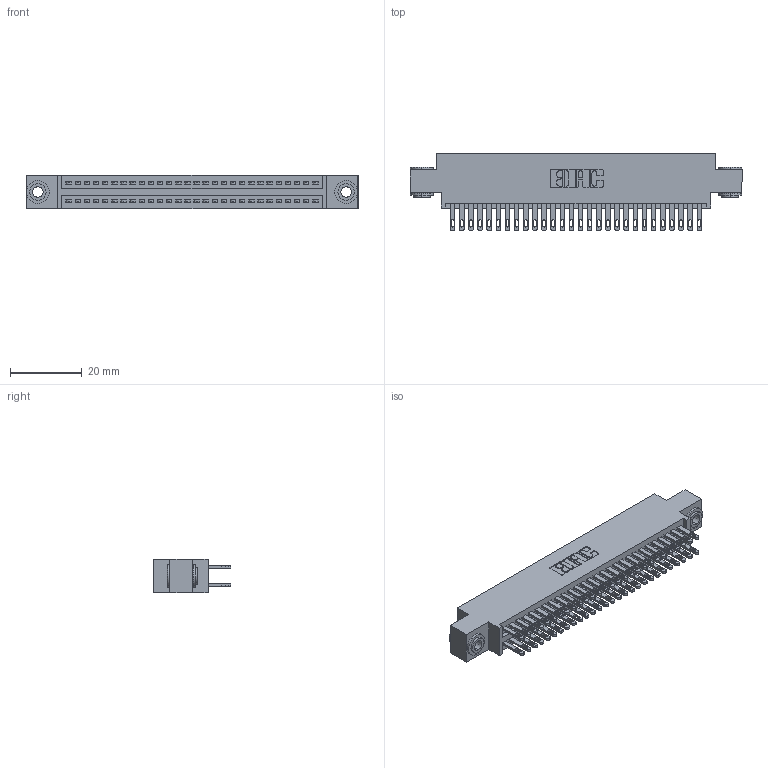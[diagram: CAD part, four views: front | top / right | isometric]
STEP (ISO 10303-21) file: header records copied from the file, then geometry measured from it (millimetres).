
FILE_DESCRIPTION (( 'STEP AP203' ), '1' );
FILE_NAME ('895-056-500-803.STEP', '2020-09-27T16:11:26', ( '' ), ( '' ), 'SwSTEP 2.0', 'SolidWorks 2020', '' );
FILE_SCHEMA (( 'CONFIG_CONTROL_DESIGN' ));
Length unit declared in the file: inch
Products named in the file (4): 345-292-001_345-293-100; 895-056-500-803; 845 Part_0.170 Offset - 0.156 Dia-TH; 345-250-002_345-250-002-102
Assembly tree (59 placements, depth 2):
  895-056-500-803
    845 Part_0.170 Offset - 0.156 Dia-TH
    345-292-001_345-293-100  x56
    345-250-002_345-250-002-102  x2
Bounding box: 92.33 x 21.51 x 9.4 mm (x, y, z)
Volume: 8916.1 mm3; surface area: 13827.9 mm2
Topology: 59 solids, 59 shells, 2744 faces, 8325 edges, 5546 vertices
Faces by surface type: plane 1606, cylinder 1130, cone 8
Entity records: 24566 total; most frequent: CARTESIAN_POINT 4107, ORIENTED_EDGE 4034, DIRECTION 3671, EDGE_CURVE 2017, LINE 1745, VECTOR 1745, VERTEX_POINT 1342, AXIS2_PLACEMENT_3D 963
